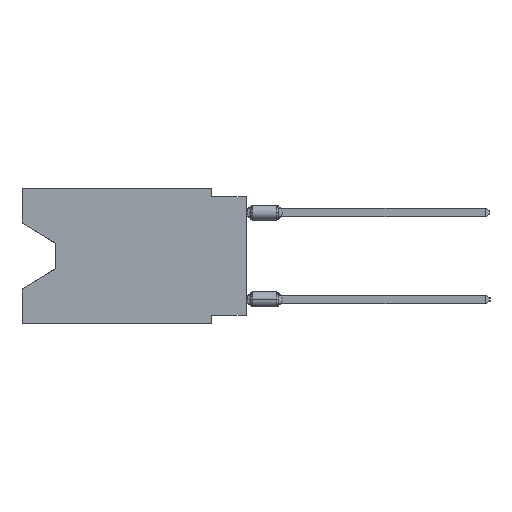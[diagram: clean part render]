
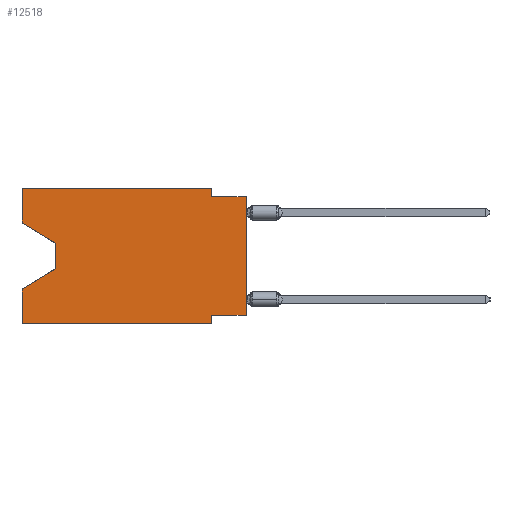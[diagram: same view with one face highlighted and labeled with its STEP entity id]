
A CAD part, left-side view. The second image highlights one B-rep face of the part: STEP entity #12518.
In plain terms, the highlighted planar face has unit normal (-1, 0, 0).
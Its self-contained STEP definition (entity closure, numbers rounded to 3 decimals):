
#464 = VECTOR ( 'NONE', #27070, 1000. ) ;
#1013 = VERTEX_POINT ( 'NONE', #9975 ) ;
#1605 = LINE ( 'NONE', #13699, #38834 ) ;
#2930 = DIRECTION ( 'NONE',  ( 0., -1., 0. ) ) ;
#3531 = EDGE_CURVE ( 'NONE', #44394, #44225, #39198, .T. ) ;
#5148 = CARTESIAN_POINT ( 'NONE',  ( 0., 2.54, -9.271 ) ) ;
#6006 = VERTEX_POINT ( 'NONE', #47462 ) ;
#6705 = CARTESIAN_POINT ( 'NONE',  ( 0., 13.97, -4.013 ) ) ;
#6802 = CARTESIAN_POINT ( 'NONE',  ( 0., 13.97, -5.893 ) ) ;
#7186 = ORIENTED_EDGE ( 'NONE', *, *, #27417, .F. ) ;
#7561 = CARTESIAN_POINT ( 'NONE',  ( 0., 16.383, -9.906 ) ) ;
#8585 = VERTEX_POINT ( 'NONE', #44671 ) ;
#9358 = VECTOR ( 'NONE', #14857, 1000. ) ;
#9602 = EDGE_CURVE ( 'NONE', #44225, #37224, #42970, .T. ) ;
#9975 = CARTESIAN_POINT ( 'NONE',  ( 0., 0., -0.635 ) ) ;
#10651 = CARTESIAN_POINT ( 'NONE',  ( 0., 16.383, 0. ) ) ;
#10731 = ORIENTED_EDGE ( 'NONE', *, *, #11528, .F. ) ;
#10960 = EDGE_CURVE ( 'NONE', #40003, #6006, #31714, .T. ) ;
#11528 = EDGE_CURVE ( 'NONE', #46538, #49330, #15201, .T. ) ;
#11813 = VECTOR ( 'NONE', #35810, 1000. ) ;
#12518 = ADVANCED_FACE ( 'NONE', ( #13760 ), #49473, .F. ) ;
#12658 = ORIENTED_EDGE ( 'NONE', *, *, #9602, .T. ) ;
#13490 = VECTOR ( 'NONE', #23670, 1000. ) ;
#13662 = ORIENTED_EDGE ( 'NONE', *, *, #32985, .T. ) ;
#13699 = CARTESIAN_POINT ( 'NONE',  ( 0., 16.383, 0. ) ) ;
#13760 = FACE_OUTER_BOUND ( 'NONE', #50086, .T. ) ;
#14254 = DIRECTION ( 'NONE',  ( 0., 0., -1. ) ) ;
#14456 = DIRECTION ( 'NONE',  ( 0., 0., 1. ) ) ;
#14857 = DIRECTION ( 'NONE',  ( 0., 0., -1. ) ) ;
#15002 = VECTOR ( 'NONE', #44742, 1000. ) ;
#15201 = LINE ( 'NONE', #31387, #44652 ) ;
#15488 = DIRECTION ( 'NONE',  ( 0., 0., -1. ) ) ;
#15763 = ORIENTED_EDGE ( 'NONE', *, *, #29508, .T. ) ;
#17945 = CARTESIAN_POINT ( 'NONE',  ( 0., 2.54, -9.906 ) ) ;
#18678 = VECTOR ( 'NONE', #27642, 1000. ) ;
#19234 = CARTESIAN_POINT ( 'NONE',  ( 0., 2.54, 0. ) ) ;
#19686 = CARTESIAN_POINT ( 'NONE',  ( 0., 16.383, -2.546 ) ) ;
#19699 = CARTESIAN_POINT ( 'NONE',  ( 0., 0., -9.271 ) ) ;
#20114 = CARTESIAN_POINT ( 'NONE',  ( 0., 16.383, 0. ) ) ;
#20458 = EDGE_CURVE ( 'NONE', #42359, #46538, #24037, .T. ) ;
#22545 = EDGE_CURVE ( 'NONE', #40398, #46212, #42249, .T. ) ;
#22631 = ORIENTED_EDGE ( 'NONE', *, *, #22545, .F. ) ;
#22696 = ORIENTED_EDGE ( 'NONE', *, *, #47316, .F. ) ;
#23168 = CARTESIAN_POINT ( 'NONE',  ( 0., 2.54, 0. ) ) ;
#23670 = DIRECTION ( 'NONE',  ( 0., 0.855, -0.519 ) ) ;
#24037 = LINE ( 'NONE', #19699, #37519 ) ;
#24261 = ORIENTED_EDGE ( 'NONE', *, *, #24534, .F. ) ;
#24534 = EDGE_CURVE ( 'NONE', #8585, #1013, #29063, .T. ) ;
#24546 = ORIENTED_EDGE ( 'NONE', *, *, #41467, .T. ) ;
#25578 = CARTESIAN_POINT ( 'NONE',  ( 0., 16.383, 0. ) ) ;
#27070 = DIRECTION ( 'NONE',  ( 0., 0., 1. ) ) ;
#27417 = EDGE_CURVE ( 'NONE', #46212, #8585, #46475, .T. ) ;
#27528 = LINE ( 'NONE', #43201, #13490 ) ;
#27642 = DIRECTION ( 'NONE',  ( 0., -0.855, -0.519 ) ) ;
#27899 = DIRECTION ( 'NONE',  ( 0., 1., 0. ) ) ;
#27970 = CARTESIAN_POINT ( 'NONE',  ( 0., 16.383, -9.906 ) ) ;
#28482 = LINE ( 'NONE', #27970, #40813 ) ;
#28571 = CARTESIAN_POINT ( 'NONE',  ( 0., 0., -0.635 ) ) ;
#28906 = VECTOR ( 'NONE', #15488, 1000. ) ;
#29063 = LINE ( 'NONE', #28571, #15002 ) ;
#29173 = DIRECTION ( 'NONE',  ( 1., 0., 0. ) ) ;
#29508 = EDGE_CURVE ( 'NONE', #37224, #6006, #27528, .T. ) ;
#30883 = DIRECTION ( 'NONE',  ( 0., 0., -1. ) ) ;
#31180 = LINE ( 'NONE', #43749, #464 ) ;
#31387 = CARTESIAN_POINT ( 'NONE',  ( 0., 2.54, -9.906 ) ) ;
#31714 = LINE ( 'NONE', #47399, #11813 ) ;
#32985 = EDGE_CURVE ( 'NONE', #40003, #49330, #28482, .T. ) ;
#34156 = ORIENTED_EDGE ( 'NONE', *, *, #3531, .T. ) ;
#35810 = DIRECTION ( 'NONE',  ( 0., 0., 1. ) ) ;
#37224 = VERTEX_POINT ( 'NONE', #6802 ) ;
#37519 = VECTOR ( 'NONE', #27899, 1000. ) ;
#37827 = VECTOR ( 'NONE', #2930, 1000. ) ;
#38834 = VECTOR ( 'NONE', #14456, 1000. ) ;
#39198 = LINE ( 'NONE', #19686, #18678 ) ;
#39303 = ORIENTED_EDGE ( 'NONE', *, *, #20458, .F. ) ;
#39523 = CARTESIAN_POINT ( 'NONE',  ( 0., 16.383, -2.546 ) ) ;
#39962 = CARTESIAN_POINT ( 'NONE',  ( 0., 0., -9.271 ) ) ;
#40003 = VERTEX_POINT ( 'NONE', #7561 ) ;
#40398 = VERTEX_POINT ( 'NONE', #20114 ) ;
#40813 = VECTOR ( 'NONE', #49222, 1000. ) ;
#41467 = EDGE_CURVE ( 'NONE', #42359, #1013, #31180, .T. ) ;
#42249 = LINE ( 'NONE', #25578, #37827 ) ;
#42359 = VERTEX_POINT ( 'NONE', #39962 ) ;
#42970 = LINE ( 'NONE', #50708, #28906 ) ;
#43201 = CARTESIAN_POINT ( 'NONE',  ( 0., 13.97, -5.893 ) ) ;
#43749 = CARTESIAN_POINT ( 'NONE',  ( 0., 0., 0. ) ) ;
#43838 = AXIS2_PLACEMENT_3D ( 'NONE', #10651, #29173, #14254 ) ;
#44225 = VERTEX_POINT ( 'NONE', #6705 ) ;
#44394 = VERTEX_POINT ( 'NONE', #39523 ) ;
#44652 = VECTOR ( 'NONE', #30883, 1000. ) ;
#44671 = CARTESIAN_POINT ( 'NONE',  ( 0., 2.54, -0.635 ) ) ;
#44742 = DIRECTION ( 'NONE',  ( 0., -1., 0. ) ) ;
#46212 = VERTEX_POINT ( 'NONE', #23168 ) ;
#46475 = LINE ( 'NONE', #19234, #9358 ) ;
#46538 = VERTEX_POINT ( 'NONE', #5148 ) ;
#47316 = EDGE_CURVE ( 'NONE', #44394, #40398, #1605, .T. ) ;
#47399 = CARTESIAN_POINT ( 'NONE',  ( 0., 16.383, 0. ) ) ;
#47462 = CARTESIAN_POINT ( 'NONE',  ( 0., 16.383, -7.36 ) ) ;
#48322 = ORIENTED_EDGE ( 'NONE', *, *, #10960, .F. ) ;
#49222 = DIRECTION ( 'NONE',  ( 0., -1., 0. ) ) ;
#49330 = VERTEX_POINT ( 'NONE', #17945 ) ;
#49473 = PLANE ( 'NONE',  #43838 ) ;
#50086 = EDGE_LOOP ( 'NONE', ( #34156, #12658, #15763, #48322, #13662, #10731, #39303, #24546, #24261, #7186, #22631, #22696 ) ) ;
#50708 = CARTESIAN_POINT ( 'NONE',  ( 0., 13.97, -4.013 ) ) ;
